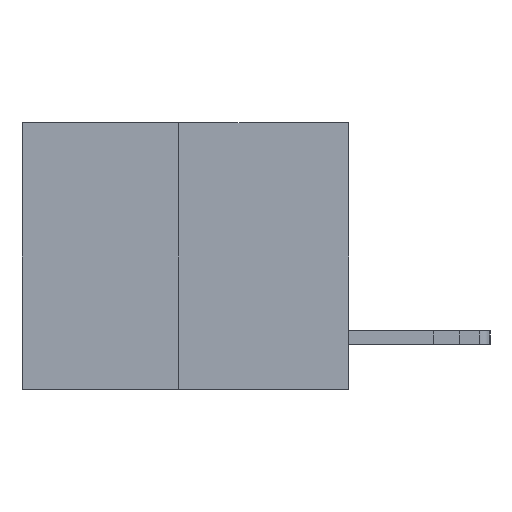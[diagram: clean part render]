
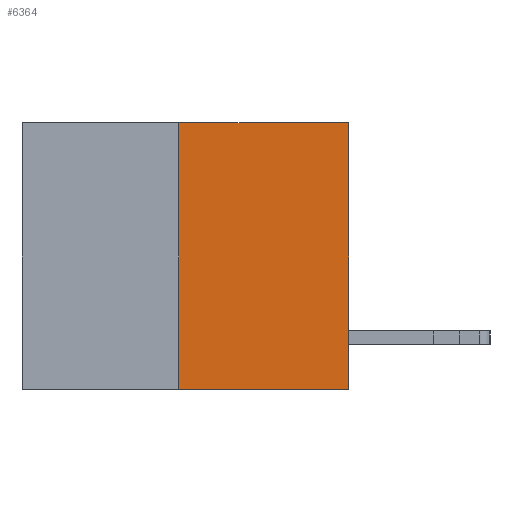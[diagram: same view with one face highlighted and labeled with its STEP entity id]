
A CAD part, left-side view. The second image highlights one B-rep face of the part: STEP entity #6364.
In plain terms, the highlighted planar face has unit normal (-1, 0, 0).
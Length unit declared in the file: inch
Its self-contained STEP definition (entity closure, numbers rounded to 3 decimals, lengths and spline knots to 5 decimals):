
#400 = LINE ( 'NONE', #12453, #22517 ) ;
#1039 = EDGE_CURVE ( 'NONE', #22902, #16213, #9191, .T. ) ;
#1370 = DIRECTION ( 'NONE',  ( 0., 0., -1. ) ) ;
#1627 = VERTEX_POINT ( 'NONE', #22534 ) ;
#2103 = CARTESIAN_POINT ( 'NONE',  ( 0., 0., 0. ) ) ;
#2475 = VECTOR ( 'NONE', #17557, 39.37008 ) ;
#2892 = DIRECTION ( 'NONE',  ( 0., 0., 1. ) ) ;
#2922 = EDGE_CURVE ( 'NONE', #11340, #16213, #13319, .T. ) ;
#3203 = PLANE ( 'NONE',  #5068 ) ;
#4340 = CARTESIAN_POINT ( 'NONE',  ( 0., 0., 0. ) ) ;
#5068 = AXIS2_PLACEMENT_3D ( 'NONE', #23862, #10703, #1370 ) ;
#6364 = ADVANCED_FACE ( 'NONE', ( #21867 ), #3203, .F. ) ;
#6751 = ORIENTED_EDGE ( 'NONE', *, *, #1039, .F. ) ;
#6875 = VECTOR ( 'NONE', #15486, 39.37008 ) ;
#8632 = EDGE_CURVE ( 'NONE', #1627, #11340, #8879, .T. ) ;
#8794 = EDGE_LOOP ( 'NONE', ( #9340, #22142, #21595, #6751 ) ) ;
#8879 = LINE ( 'NONE', #20395, #21913 ) ;
#9191 = LINE ( 'NONE', #17906, #2475 ) ;
#9340 = ORIENTED_EDGE ( 'NONE', *, *, #18310, .F. ) ;
#10703 = DIRECTION ( 'NONE',  ( 1., 0., 0. ) ) ;
#11340 = VERTEX_POINT ( 'NONE', #14883 ) ;
#12453 = CARTESIAN_POINT ( 'NONE',  ( 0., 0.312, -0.49 ) ) ;
#13319 = LINE ( 'NONE', #4340, #6875 ) ;
#14883 = CARTESIAN_POINT ( 'NONE',  ( 0., 0., -0.49 ) ) ;
#15486 = DIRECTION ( 'NONE',  ( 0., 0., 1. ) ) ;
#16213 = VERTEX_POINT ( 'NONE', #2103 ) ;
#17102 = DIRECTION ( 'NONE',  ( 0., -1., 0. ) ) ;
#17557 = DIRECTION ( 'NONE',  ( 0., -1., 0. ) ) ;
#17678 = CARTESIAN_POINT ( 'NONE',  ( 0., 0.312, 0. ) ) ;
#17906 = CARTESIAN_POINT ( 'NONE',  ( 0., 0.6, 0. ) ) ;
#18310 = EDGE_CURVE ( 'NONE', #1627, #22902, #400, .T. ) ;
#20395 = CARTESIAN_POINT ( 'NONE',  ( 0., 0.6, -0.49 ) ) ;
#21595 = ORIENTED_EDGE ( 'NONE', *, *, #2922, .T. ) ;
#21867 = FACE_OUTER_BOUND ( 'NONE', #8794, .T. ) ;
#21913 = VECTOR ( 'NONE', #17102, 39.37008 ) ;
#22142 = ORIENTED_EDGE ( 'NONE', *, *, #8632, .T. ) ;
#22517 = VECTOR ( 'NONE', #2892, 39.37008 ) ;
#22534 = CARTESIAN_POINT ( 'NONE',  ( 0., 0.312, -0.49 ) ) ;
#22902 = VERTEX_POINT ( 'NONE', #17678 ) ;
#23862 = CARTESIAN_POINT ( 'NONE',  ( 0., 0.6, 0. ) ) ;
